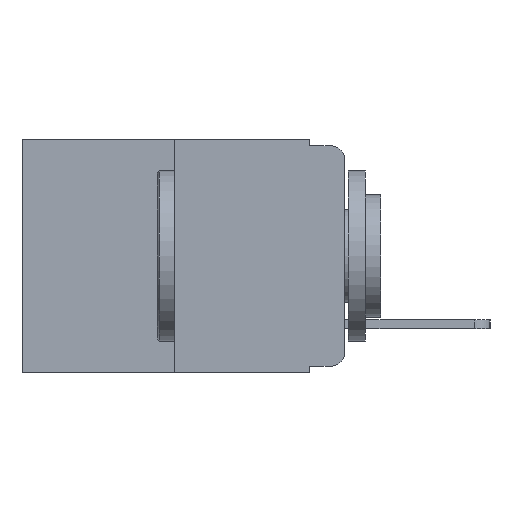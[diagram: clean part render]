
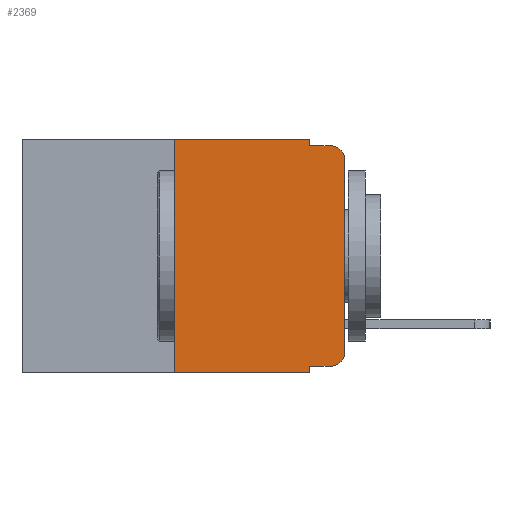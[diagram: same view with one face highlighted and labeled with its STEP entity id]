
A CAD part, left-side view. The second image highlights one B-rep face of the part: STEP entity #2369.
In plain terms, the highlighted planar face has unit normal (-1, 0, 0).
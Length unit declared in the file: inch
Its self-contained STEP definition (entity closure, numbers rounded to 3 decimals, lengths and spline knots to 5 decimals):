
#927 = CARTESIAN_POINT ( 'NONE',  ( 0., 0.051, 0. ) ) ;
#1394 = ORIENTED_EDGE ( 'NONE', *, *, #8914, .F. ) ;
#1842 = CARTESIAN_POINT ( 'NONE',  ( 0., 0.02, -0.03 ) ) ;
#2223 = EDGE_CURVE ( 'NONE', #4421, #19952, #4530, .T. ) ;
#2369 = ADVANCED_FACE ( 'NONE', ( #6318 ), #14600, .F. ) ;
#2406 = ORIENTED_EDGE ( 'NONE', *, *, #18163, .F. ) ;
#2663 = LINE ( 'NONE', #12364, #18498 ) ;
#2816 = CARTESIAN_POINT ( 'NONE',  ( 0., 0.051, 0. ) ) ;
#3106 = VERTEX_POINT ( 'NONE', #3617 ) ;
#3278 = EDGE_LOOP ( 'NONE', ( #3882, #11590, #6102, #6030, #4299, #2406, #6203, #1394, #15328, #15427 ) ) ;
#3400 = AXIS2_PLACEMENT_3D ( 'NONE', #19920, #9546, #17512 ) ;
#3562 = DIRECTION ( 'NONE',  ( 0., 0., -1. ) ) ;
#3617 = CARTESIAN_POINT ( 'NONE',  ( 0., 0.25, 0. ) ) ;
#3882 = ORIENTED_EDGE ( 'NONE', *, *, #13617, .T. ) ;
#4254 = DIRECTION ( 'NONE',  ( 0., -1., 0. ) ) ;
#4299 = ORIENTED_EDGE ( 'NONE', *, *, #8734, .F. ) ;
#4421 = VERTEX_POINT ( 'NONE', #15767 ) ;
#4494 = LINE ( 'NONE', #19041, #16514 ) ;
#4530 = CIRCLE ( 'NONE', #3400, 0.02 ) ;
#5055 = CARTESIAN_POINT ( 'NONE',  ( 0., 0.473, 0. ) ) ;
#5233 = EDGE_CURVE ( 'NONE', #7715, #7162, #20606, .T. ) ;
#5288 = VECTOR ( 'NONE', #20219, 39.37008 ) ;
#6025 = VECTOR ( 'NONE', #11554, 39.37008 ) ;
#6030 = ORIENTED_EDGE ( 'NONE', *, *, #5233, .F. ) ;
#6102 = ORIENTED_EDGE ( 'NONE', *, *, #9550, .F. ) ;
#6203 = ORIENTED_EDGE ( 'NONE', *, *, #18077, .T. ) ;
#6318 = FACE_OUTER_BOUND ( 'NONE', #3278, .T. ) ;
#7162 = VERTEX_POINT ( 'NONE', #7517 ) ;
#7517 = CARTESIAN_POINT ( 'NONE',  ( 0., 0.051, -0.01 ) ) ;
#7619 = LINE ( 'NONE', #15271, #8142 ) ;
#7690 = VERTEX_POINT ( 'NONE', #18500 ) ;
#7715 = VERTEX_POINT ( 'NONE', #2816 ) ;
#7842 = EDGE_CURVE ( 'NONE', #7690, #4421, #7619, .T. ) ;
#8096 = VECTOR ( 'NONE', #17367, 39.37008 ) ;
#8135 = CARTESIAN_POINT ( 'NONE',  ( 0., 0.473, 0. ) ) ;
#8142 = VECTOR ( 'NONE', #4254, 39.37008 ) ;
#8494 = DIRECTION ( 'NONE',  ( 0., 0., -1. ) ) ;
#8734 = EDGE_CURVE ( 'NONE', #3106, #7715, #20313, .T. ) ;
#8759 = VERTEX_POINT ( 'NONE', #9760 ) ;
#8914 = EDGE_CURVE ( 'NONE', #7690, #8759, #14333, .T. ) ;
#9546 = DIRECTION ( 'NONE',  ( -1., 0., 0. ) ) ;
#9550 = EDGE_CURVE ( 'NONE', #7162, #13758, #17755, .T. ) ;
#9625 = CARTESIAN_POINT ( 'NONE',  ( 0., 0.02, -0.01 ) ) ;
#9760 = CARTESIAN_POINT ( 'NONE',  ( 0., 0.051, -0.343 ) ) ;
#10033 = CARTESIAN_POINT ( 'NONE',  ( 0., 0.051, 0. ) ) ;
#10570 = EDGE_CURVE ( 'NONE', #13778, #13758, #18601, .T. ) ;
#11139 = CARTESIAN_POINT ( 'NONE',  ( 0., 0.051, -0.01 ) ) ;
#11389 = DIRECTION ( 'NONE',  ( 0., -1., 0. ) ) ;
#11554 = DIRECTION ( 'NONE',  ( 0., 0., -1. ) ) ;
#11590 = ORIENTED_EDGE ( 'NONE', *, *, #10570, .T. ) ;
#12364 = CARTESIAN_POINT ( 'NONE',  ( 0., 0., 0. ) ) ;
#12626 = AXIS2_PLACEMENT_3D ( 'NONE', #5055, #15625, #8494 ) ;
#13064 = DIRECTION ( 'NONE',  ( -1., 0., 0. ) ) ;
#13617 = EDGE_CURVE ( 'NONE', #19952, #13778, #2663, .T. ) ;
#13758 = VERTEX_POINT ( 'NONE', #9625 ) ;
#13778 = VERTEX_POINT ( 'NONE', #18886 ) ;
#14298 = DIRECTION ( 'NONE',  ( 0., 0., 1. ) ) ;
#14333 = LINE ( 'NONE', #10033, #6025 ) ;
#14495 = CARTESIAN_POINT ( 'NONE',  ( 0., 0.25, -0.343 ) ) ;
#14586 = VECTOR ( 'NONE', #14298, 39.37008 ) ;
#14600 = PLANE ( 'NONE',  #12626 ) ;
#15063 = LINE ( 'NONE', #17721, #14586 ) ;
#15254 = CARTESIAN_POINT ( 'NONE',  ( 0., 0., -0.313 ) ) ;
#15271 = CARTESIAN_POINT ( 'NONE',  ( 0., 0.051, -0.333 ) ) ;
#15328 = ORIENTED_EDGE ( 'NONE', *, *, #7842, .T. ) ;
#15393 = DIRECTION ( 'NONE',  ( 0., 0., -1. ) ) ;
#15427 = ORIENTED_EDGE ( 'NONE', *, *, #2223, .T. ) ;
#15463 = DIRECTION ( 'NONE',  ( 0., 0., 1. ) ) ;
#15501 = AXIS2_PLACEMENT_3D ( 'NONE', #1842, #13064, #3562 ) ;
#15625 = DIRECTION ( 'NONE',  ( 1., 0., 0. ) ) ;
#15767 = CARTESIAN_POINT ( 'NONE',  ( 0., 0.02, -0.333 ) ) ;
#16514 = VECTOR ( 'NONE', #11389, 39.37008 ) ;
#17367 = DIRECTION ( 'NONE',  ( 0., -1., 0. ) ) ;
#17512 = DIRECTION ( 'NONE',  ( 0., 0., -1. ) ) ;
#17721 = CARTESIAN_POINT ( 'NONE',  ( 0., 0.25, 0. ) ) ;
#17755 = LINE ( 'NONE', #11139, #5288 ) ;
#18077 = EDGE_CURVE ( 'NONE', #18273, #8759, #4494, .T. ) ;
#18163 = EDGE_CURVE ( 'NONE', #18273, #3106, #15063, .T. ) ;
#18273 = VERTEX_POINT ( 'NONE', #14495 ) ;
#18498 = VECTOR ( 'NONE', #15463, 39.37008 ) ;
#18500 = CARTESIAN_POINT ( 'NONE',  ( 0., 0.051, -0.333 ) ) ;
#18601 = CIRCLE ( 'NONE', #15501, 0.02 ) ;
#18886 = CARTESIAN_POINT ( 'NONE',  ( 0., 0., -0.03 ) ) ;
#19041 = CARTESIAN_POINT ( 'NONE',  ( 0., 0.473, -0.343 ) ) ;
#19920 = CARTESIAN_POINT ( 'NONE',  ( 0., 0.02, -0.313 ) ) ;
#19952 = VERTEX_POINT ( 'NONE', #15254 ) ;
#20141 = VECTOR ( 'NONE', #15393, 39.37008 ) ;
#20219 = DIRECTION ( 'NONE',  ( 0., -1., 0. ) ) ;
#20313 = LINE ( 'NONE', #8135, #8096 ) ;
#20606 = LINE ( 'NONE', #927, #20141 ) ;
